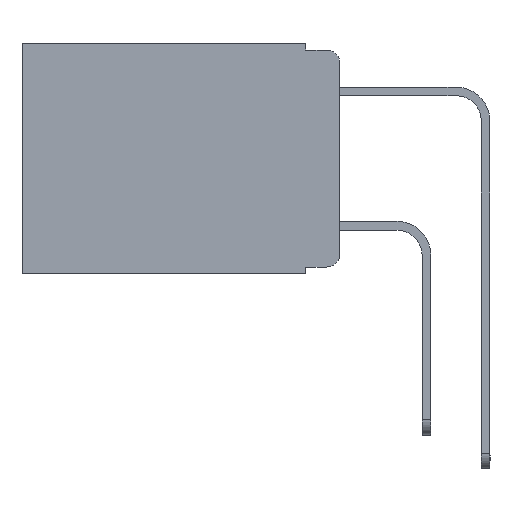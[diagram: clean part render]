
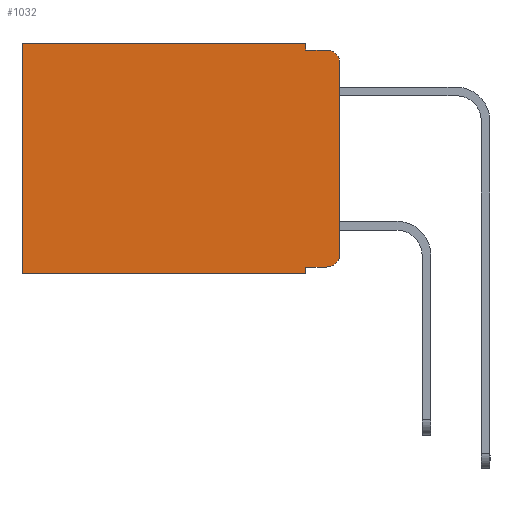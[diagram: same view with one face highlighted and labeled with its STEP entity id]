
A CAD part, left-side view. The second image highlights one B-rep face of the part: STEP entity #1032.
In plain terms, the highlighted planar face has unit normal (-1, 0, 0).
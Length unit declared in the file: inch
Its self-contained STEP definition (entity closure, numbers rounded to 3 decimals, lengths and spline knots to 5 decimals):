
#149 = CARTESIAN_POINT ( 'NONE',  ( 0.298, 0.02, -0.01 ) ) ;
#673 = CARTESIAN_POINT ( 'NONE',  ( 0.298, 0.473, -0.343 ) ) ;
#1032 = ADVANCED_FACE ( 'NONE', ( #24442 ), #8586, .F. ) ;
#1318 = VERTEX_POINT ( 'NONE', #149 ) ;
#1454 = CARTESIAN_POINT ( 'NONE',  ( 0.298, 0.02, -0.333 ) ) ;
#1692 = VERTEX_POINT ( 'NONE', #21437 ) ;
#1970 = LINE ( 'NONE', #13726, #21339 ) ;
#2170 = ORIENTED_EDGE ( 'NONE', *, *, #2407, .T. ) ;
#2407 = EDGE_CURVE ( 'NONE', #24323, #20883, #14803, .T. ) ;
#2532 = DIRECTION ( 'NONE',  ( 0., 0., -1. ) ) ;
#2853 = CARTESIAN_POINT ( 'NONE',  ( 0.298, 0., 0. ) ) ;
#3544 = ORIENTED_EDGE ( 'NONE', *, *, #17428, .F. ) ;
#4233 = EDGE_CURVE ( 'NONE', #23847, #19935, #4475, .T. ) ;
#4308 = ORIENTED_EDGE ( 'NONE', *, *, #7393, .T. ) ;
#4475 = LINE ( 'NONE', #18550, #21728 ) ;
#5097 = EDGE_CURVE ( 'NONE', #5779, #20883, #20545, .T. ) ;
#5104 = DIRECTION ( 'NONE',  ( -1., 0., 0. ) ) ;
#5455 = AXIS2_PLACEMENT_3D ( 'NONE', #24434, #12686, #19014 ) ;
#5476 = CARTESIAN_POINT ( 'NONE',  ( 0.298, 0.473, 0. ) ) ;
#5779 = VERTEX_POINT ( 'NONE', #23685 ) ;
#5950 = DIRECTION ( 'NONE',  ( 0., 0., -1. ) ) ;
#6934 = VECTOR ( 'NONE', #23905, 39.37008 ) ;
#7393 = EDGE_CURVE ( 'NONE', #1692, #24323, #1970, .T. ) ;
#8586 = PLANE ( 'NONE',  #25517 ) ;
#9163 = EDGE_CURVE ( 'NONE', #19935, #1318, #17855, .T. ) ;
#9257 = VERTEX_POINT ( 'NONE', #673 ) ;
#9496 = CARTESIAN_POINT ( 'NONE',  ( 0.298, 0., 0. ) ) ;
#9581 = VERTEX_POINT ( 'NONE', #10083 ) ;
#10083 = CARTESIAN_POINT ( 'NONE',  ( 0.298, 0.051, -0.343 ) ) ;
#10288 = VECTOR ( 'NONE', #11804, 39.37008 ) ;
#10444 = ORIENTED_EDGE ( 'NONE', *, *, #11832, .T. ) ;
#10616 = VECTOR ( 'NONE', #12355, 39.37008 ) ;
#10995 = VECTOR ( 'NONE', #23228, 39.37008 ) ;
#11187 = ORIENTED_EDGE ( 'NONE', *, *, #4233, .F. ) ;
#11320 = LINE ( 'NONE', #9496, #13244 ) ;
#11417 = CARTESIAN_POINT ( 'NONE',  ( 0.298, 0.02, -0.313 ) ) ;
#11804 = DIRECTION ( 'NONE',  ( 0., -1., 0. ) ) ;
#11832 = EDGE_CURVE ( 'NONE', #23847, #14871, #11320, .T. ) ;
#11866 = CARTESIAN_POINT ( 'NONE',  ( 0.298, 0., -0.343 ) ) ;
#12183 = CARTESIAN_POINT ( 'NONE',  ( 0.298, 0., 0. ) ) ;
#12355 = DIRECTION ( 'NONE',  ( 0., 1., 0. ) ) ;
#12560 = DIRECTION ( 'NONE',  ( 1., 0., 0. ) ) ;
#12686 = DIRECTION ( 'NONE',  ( -1., 0., 0. ) ) ;
#13244 = VECTOR ( 'NONE', #21234, 39.37008 ) ;
#13666 = CARTESIAN_POINT ( 'NONE',  ( 0.298, 0.051, -0.01 ) ) ;
#13726 = CARTESIAN_POINT ( 'NONE',  ( 0.298, 0.051, -0.333 ) ) ;
#13862 = VECTOR ( 'NONE', #5950, 39.37008 ) ;
#14049 = ORIENTED_EDGE ( 'NONE', *, *, #5097, .F. ) ;
#14052 = CARTESIAN_POINT ( 'NONE',  ( 0.298, 0.051, 0. ) ) ;
#14088 = EDGE_CURVE ( 'NONE', #14871, #9257, #15854, .T. ) ;
#14803 = CIRCLE ( 'NONE', #18101, 0.02 ) ;
#14871 = VERTEX_POINT ( 'NONE', #5476 ) ;
#15478 = CARTESIAN_POINT ( 'NONE',  ( 0.298, 0.473, 0. ) ) ;
#15717 = LINE ( 'NONE', #25290, #10995 ) ;
#15818 = ORIENTED_EDGE ( 'NONE', *, *, #19985, .F. ) ;
#15854 = LINE ( 'NONE', #15478, #13862 ) ;
#16564 = CIRCLE ( 'NONE', #5455, 0.02 ) ;
#17158 = ORIENTED_EDGE ( 'NONE', *, *, #25385, .T. ) ;
#17428 = EDGE_CURVE ( 'NONE', #9581, #9257, #23848, .T. ) ;
#17589 = DIRECTION ( 'NONE',  ( 0., -1., 0. ) ) ;
#17855 = LINE ( 'NONE', #25348, #10288 ) ;
#18101 = AXIS2_PLACEMENT_3D ( 'NONE', #11417, #5104, #18774 ) ;
#18550 = CARTESIAN_POINT ( 'NONE',  ( 0.298, 0.051, 0. ) ) ;
#18774 = DIRECTION ( 'NONE',  ( 0., 0., -1. ) ) ;
#19014 = DIRECTION ( 'NONE',  ( 0., 0., -1. ) ) ;
#19935 = VERTEX_POINT ( 'NONE', #13666 ) ;
#19985 = EDGE_CURVE ( 'NONE', #1692, #9581, #15717, .T. ) ;
#20242 = EDGE_LOOP ( 'NONE', ( #14049, #17158, #24115, #11187, #10444, #24915, #3544, #15818, #4308, #2170 ) ) ;
#20265 = CARTESIAN_POINT ( 'NONE',  ( 0.298, 0., -0.313 ) ) ;
#20545 = LINE ( 'NONE', #2853, #6934 ) ;
#20883 = VERTEX_POINT ( 'NONE', #20265 ) ;
#21234 = DIRECTION ( 'NONE',  ( 0., 1., 0. ) ) ;
#21339 = VECTOR ( 'NONE', #17589, 39.37008 ) ;
#21437 = CARTESIAN_POINT ( 'NONE',  ( 0.298, 0.051, -0.333 ) ) ;
#21728 = VECTOR ( 'NONE', #2532, 39.37008 ) ;
#22504 = DIRECTION ( 'NONE',  ( 0., 0., -1. ) ) ;
#23228 = DIRECTION ( 'NONE',  ( 0., 0., -1. ) ) ;
#23685 = CARTESIAN_POINT ( 'NONE',  ( 0.298, 0., -0.03 ) ) ;
#23847 = VERTEX_POINT ( 'NONE', #14052 ) ;
#23848 = LINE ( 'NONE', #11866, #10616 ) ;
#23905 = DIRECTION ( 'NONE',  ( 0., 0., -1. ) ) ;
#24115 = ORIENTED_EDGE ( 'NONE', *, *, #9163, .F. ) ;
#24323 = VERTEX_POINT ( 'NONE', #1454 ) ;
#24434 = CARTESIAN_POINT ( 'NONE',  ( 0.298, 0.02, -0.03 ) ) ;
#24442 = FACE_OUTER_BOUND ( 'NONE', #20242, .T. ) ;
#24915 = ORIENTED_EDGE ( 'NONE', *, *, #14088, .T. ) ;
#25290 = CARTESIAN_POINT ( 'NONE',  ( 0.298, 0.051, 0. ) ) ;
#25348 = CARTESIAN_POINT ( 'NONE',  ( 0.298, 0.051, -0.01 ) ) ;
#25385 = EDGE_CURVE ( 'NONE', #5779, #1318, #16564, .T. ) ;
#25517 = AXIS2_PLACEMENT_3D ( 'NONE', #12183, #12560, #22504 ) ;
